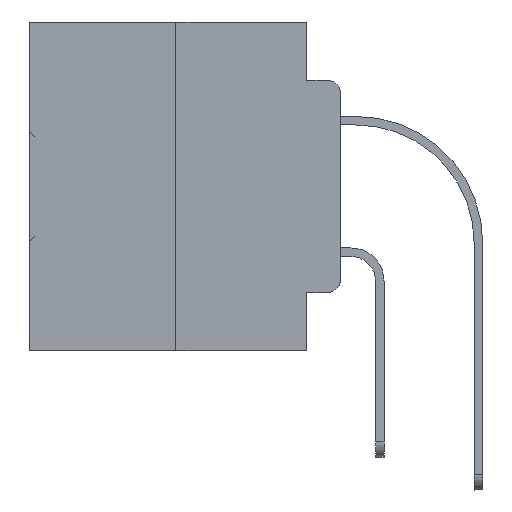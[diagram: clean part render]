
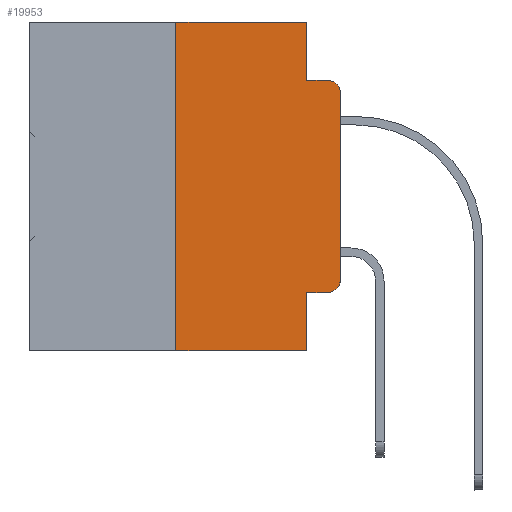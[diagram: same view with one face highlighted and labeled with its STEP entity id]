
A CAD part, left-side view. The second image highlights one B-rep face of the part: STEP entity #19953.
In plain terms, the highlighted planar face has unit normal (-1, 0, 0).
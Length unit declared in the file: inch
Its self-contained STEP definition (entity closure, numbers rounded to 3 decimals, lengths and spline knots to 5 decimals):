
#585 = CARTESIAN_POINT ( 'NONE',  ( 0., 0.25, 0. ) ) ;
#1048 = EDGE_CURVE ( 'NONE', #17663, #30844, #25938, .T. ) ;
#1100 = EDGE_LOOP ( 'NONE', ( #19456, #32186, #22204, #23993, #21045, #33664, #4785, #17897, #12862, #8905 ) ) ;
#1116 = CIRCLE ( 'NONE', #15868, 0.02 ) ;
#1735 = CARTESIAN_POINT ( 'NONE',  ( 0., 0.051, 0. ) ) ;
#1856 = EDGE_CURVE ( 'NONE', #24256, #24705, #31559, .T. ) ;
#2271 = EDGE_CURVE ( 'NONE', #17663, #33831, #6328, .T. ) ;
#3166 = CARTESIAN_POINT ( 'NONE',  ( 0., 0.473, 0. ) ) ;
#3354 = VERTEX_POINT ( 'NONE', #35005 ) ;
#3676 = DIRECTION ( 'NONE',  ( 0., 0., -1. ) ) ;
#4117 = LINE ( 'NONE', #26668, #7449 ) ;
#4249 = VECTOR ( 'NONE', #17852, 39.37008 ) ;
#4505 = CIRCLE ( 'NONE', #6869, 0.02 ) ;
#4513 = EDGE_CURVE ( 'NONE', #9235, #24256, #30823, .T. ) ;
#4785 = ORIENTED_EDGE ( 'NONE', *, *, #2271, .T. ) ;
#5281 = VECTOR ( 'NONE', #11883, 39.37008 ) ;
#5411 = VECTOR ( 'NONE', #20511, 39.37008 ) ;
#5468 = CARTESIAN_POINT ( 'NONE',  ( 0., 0.02, -0.0885 ) ) ;
#5648 = CARTESIAN_POINT ( 'NONE',  ( 0., 0.25, -0.5 ) ) ;
#6055 = DIRECTION ( 'NONE',  ( 0., -1., 0. ) ) ;
#6127 = DIRECTION ( 'NONE',  ( 0., 0., -1. ) ) ;
#6328 = LINE ( 'NONE', #29241, #25779 ) ;
#6450 = DIRECTION ( 'NONE',  ( -1., 0., 0. ) ) ;
#6492 = DIRECTION ( 'NONE',  ( 1., 0., 0. ) ) ;
#6869 = AXIS2_PLACEMENT_3D ( 'NONE', #31784, #6450, #3676 ) ;
#7449 = VECTOR ( 'NONE', #11727, 39.37008 ) ;
#7736 = DIRECTION ( 'NONE',  ( 0., 0., -1. ) ) ;
#8878 = CARTESIAN_POINT ( 'NONE',  ( 0., 0., 0. ) ) ;
#8905 = ORIENTED_EDGE ( 'NONE', *, *, #10049, .T. ) ;
#9235 = VERTEX_POINT ( 'NONE', #1735 ) ;
#9942 = VERTEX_POINT ( 'NONE', #21051 ) ;
#10049 = EDGE_CURVE ( 'NONE', #3354, #9942, #4505, .T. ) ;
#11017 = AXIS2_PLACEMENT_3D ( 'NONE', #3166, #6492, #6127 ) ;
#11727 = DIRECTION ( 'NONE',  ( 0., -1., 0. ) ) ;
#11883 = DIRECTION ( 'NONE',  ( 0., 0., 1. ) ) ;
#12128 = CARTESIAN_POINT ( 'NONE',  ( 0., 0.473, 0. ) ) ;
#12862 = ORIENTED_EDGE ( 'NONE', *, *, #19599, .T. ) ;
#13535 = CARTESIAN_POINT ( 'NONE',  ( 0., 0.051, -0.4115 ) ) ;
#13976 = EDGE_CURVE ( 'NONE', #9942, #32328, #36035, .T. ) ;
#14049 = CARTESIAN_POINT ( 'NONE',  ( 0., 0.25, 0. ) ) ;
#14226 = CARTESIAN_POINT ( 'NONE',  ( 0., 0.051, -0.5 ) ) ;
#15868 = AXIS2_PLACEMENT_3D ( 'NONE', #18712, #23549, #26670 ) ;
#15979 = DIRECTION ( 'NONE',  ( 0., 0., -1. ) ) ;
#16158 = LINE ( 'NONE', #30752, #30806 ) ;
#17596 = FACE_OUTER_BOUND ( 'NONE', #1100, .T. ) ;
#17663 = VERTEX_POINT ( 'NONE', #5648 ) ;
#17733 = CARTESIAN_POINT ( 'NONE',  ( 0., 0., -0.1085 ) ) ;
#17852 = DIRECTION ( 'NONE',  ( 0., -1., 0. ) ) ;
#17897 = ORIENTED_EDGE ( 'NONE', *, *, #31715, .F. ) ;
#18712 = CARTESIAN_POINT ( 'NONE',  ( 0., 0.02, -0.1085 ) ) ;
#19456 = ORIENTED_EDGE ( 'NONE', *, *, #13976, .T. ) ;
#19599 = EDGE_CURVE ( 'NONE', #25269, #3354, #4117, .T. ) ;
#19953 = ADVANCED_FACE ( 'NONE', ( #17596 ), #28873, .F. ) ;
#20511 = DIRECTION ( 'NONE',  ( 0., 0., 1. ) ) ;
#21045 = ORIENTED_EDGE ( 'NONE', *, *, #34585, .F. ) ;
#21051 = CARTESIAN_POINT ( 'NONE',  ( 0., 0., -0.3915 ) ) ;
#21886 = CARTESIAN_POINT ( 'NONE',  ( 0., 0.051, -0.0885 ) ) ;
#22204 = ORIENTED_EDGE ( 'NONE', *, *, #1856, .F. ) ;
#23335 = DIRECTION ( 'NONE',  ( 0., -1., 0. ) ) ;
#23549 = DIRECTION ( 'NONE',  ( -1., 0., 0. ) ) ;
#23993 = ORIENTED_EDGE ( 'NONE', *, *, #4513, .F. ) ;
#24256 = VERTEX_POINT ( 'NONE', #21886 ) ;
#24705 = VERTEX_POINT ( 'NONE', #5468 ) ;
#25269 = VERTEX_POINT ( 'NONE', #13535 ) ;
#25779 = VECTOR ( 'NONE', #23335, 39.37008 ) ;
#25938 = LINE ( 'NONE', #585, #5281 ) ;
#26501 = EDGE_CURVE ( 'NONE', #32328, #24705, #1116, .T. ) ;
#26668 = CARTESIAN_POINT ( 'NONE',  ( 0., 0.051, -0.4115 ) ) ;
#26670 = DIRECTION ( 'NONE',  ( 0., 0., -1. ) ) ;
#27010 = VECTOR ( 'NONE', #7736, 39.37008 ) ;
#27536 = VECTOR ( 'NONE', #6055, 39.37008 ) ;
#28432 = CARTESIAN_POINT ( 'NONE',  ( 0., 0.051, -0.0885 ) ) ;
#28873 = PLANE ( 'NONE',  #11017 ) ;
#29241 = CARTESIAN_POINT ( 'NONE',  ( 0., 0.473, -0.5 ) ) ;
#30100 = CARTESIAN_POINT ( 'NONE',  ( 0., 0.051, 0. ) ) ;
#30752 = CARTESIAN_POINT ( 'NONE',  ( 0., 0.051, 0. ) ) ;
#30806 = VECTOR ( 'NONE', #15979, 39.37008 ) ;
#30823 = LINE ( 'NONE', #30100, #27010 ) ;
#30844 = VERTEX_POINT ( 'NONE', #14049 ) ;
#31559 = LINE ( 'NONE', #28432, #27536 ) ;
#31715 = EDGE_CURVE ( 'NONE', #25269, #33831, #16158, .T. ) ;
#31784 = CARTESIAN_POINT ( 'NONE',  ( 0., 0.02, -0.3915 ) ) ;
#31905 = LINE ( 'NONE', #12128, #4249 ) ;
#32186 = ORIENTED_EDGE ( 'NONE', *, *, #26501, .T. ) ;
#32328 = VERTEX_POINT ( 'NONE', #17733 ) ;
#33664 = ORIENTED_EDGE ( 'NONE', *, *, #1048, .F. ) ;
#33831 = VERTEX_POINT ( 'NONE', #14226 ) ;
#34585 = EDGE_CURVE ( 'NONE', #30844, #9235, #31905, .T. ) ;
#35005 = CARTESIAN_POINT ( 'NONE',  ( 0., 0.02, -0.4115 ) ) ;
#36035 = LINE ( 'NONE', #8878, #5411 ) ;
